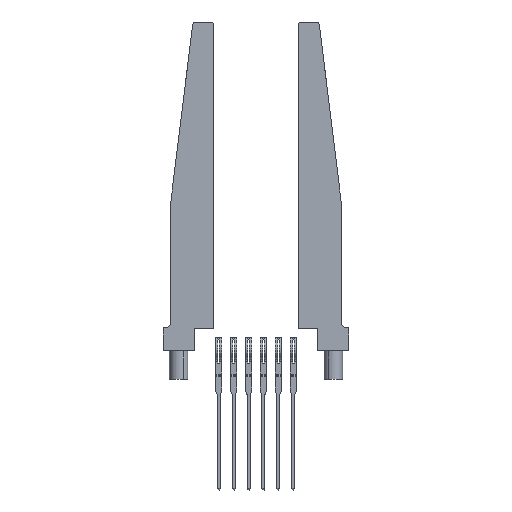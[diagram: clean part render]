
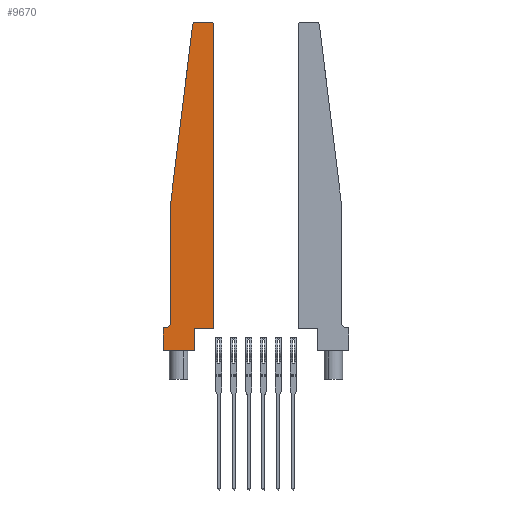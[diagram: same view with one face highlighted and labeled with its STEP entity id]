
A CAD part, top view. The second image highlights one B-rep face of the part: STEP entity #9670.
In plain terms, the highlighted planar face has unit normal (0, 0, 1).
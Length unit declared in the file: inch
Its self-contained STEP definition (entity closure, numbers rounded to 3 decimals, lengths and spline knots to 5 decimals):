
#51 = EDGE_CURVE ( 'NONE', #11635, #7275, #797, .T. ) ;
#185 = VECTOR ( 'NONE', #13633, 39.37008 ) ;
#228 = CARTESIAN_POINT ( 'NONE',  ( 0.065, 0.2375, 0.37 ) ) ;
#387 = CARTESIAN_POINT ( 'NONE',  ( 0.065, 1.25, 0.37 ) ) ;
#487 = VERTEX_POINT ( 'NONE', #6014 ) ;
#513 = DIRECTION ( 'NONE',  ( 0., 0., 1. ) ) ;
#551 = VERTEX_POINT ( 'NONE', #4396 ) ;
#700 = CARTESIAN_POINT ( 'NONE',  ( 0.015, 0.2375, 0.37 ) ) ;
#797 = LINE ( 'NONE', #8160, #4274 ) ;
#814 = ORIENTED_EDGE ( 'NONE', *, *, #6309, .T. ) ;
#1166 = CARTESIAN_POINT ( 'NONE',  ( 0.2605, 0.18, 0.37 ) ) ;
#1531 = EDGE_CURVE ( 'NONE', #5878, #4005, #7129, .T. ) ;
#1551 = EDGE_CURVE ( 'NONE', #8311, #2658, #11511, .T. ) ;
#1616 = CARTESIAN_POINT ( 'NONE',  ( 0.395, 2.75, 0.37 ) ) ;
#1831 = AXIS2_PLACEMENT_3D ( 'NONE', #700, #3854, #13475 ) ;
#1925 = DIRECTION ( 'NONE',  ( 1., 0., 0. ) ) ;
#1995 = CARTESIAN_POINT ( 'NONE',  ( 0., 0.1875, 0.37 ) ) ;
#2031 = DIRECTION ( 'NONE',  ( 1., 0., 0. ) ) ;
#2064 = FACE_OUTER_BOUND ( 'NONE', #13731, .T. ) ;
#2277 = VERTEX_POINT ( 'NONE', #7781 ) ;
#2502 = DIRECTION ( 'NONE',  ( 0., -1., 0. ) ) ;
#2549 = EDGE_CURVE ( 'NONE', #7275, #3619, #2656, .T. ) ;
#2588 = DIRECTION ( 'NONE',  ( 1., 0., 0. ) ) ;
#2656 = LINE ( 'NONE', #387, #12060 ) ;
#2658 = VERTEX_POINT ( 'NONE', #3944 ) ;
#2678 = VECTOR ( 'NONE', #10494, 39.37008 ) ;
#2684 = ORIENTED_EDGE ( 'NONE', *, *, #10316, .T. ) ;
#2731 = ORIENTED_EDGE ( 'NONE', *, *, #11652, .T. ) ;
#2940 = ORIENTED_EDGE ( 'NONE', *, *, #7992, .T. ) ;
#2974 = CARTESIAN_POINT ( 'NONE',  ( 0.25, 2.75, 0.37 ) ) ;
#3008 = VECTOR ( 'NONE', #7226, 39.37008 ) ;
#3022 = CARTESIAN_POINT ( 'NONE',  ( 0., 0., 0.37 ) ) ;
#3124 = CARTESIAN_POINT ( 'NONE',  ( 0.2605, 0.18, 0.37 ) ) ;
#3207 = ORIENTED_EDGE ( 'NONE', *, *, #13453, .T. ) ;
#3357 = LINE ( 'NONE', #1166, #5713 ) ;
#3521 = CARTESIAN_POINT ( 'NONE',  ( 0.425, 0.18, 0.37 ) ) ;
#3539 = DIRECTION ( 'NONE',  ( 0., -1., 0. ) ) ;
#3619 = VERTEX_POINT ( 'NONE', #228 ) ;
#3685 = ORIENTED_EDGE ( 'NONE', *, *, #2549, .T. ) ;
#3825 = EDGE_CURVE ( 'NONE', #9360, #8311, #7421, .T. ) ;
#3838 = CARTESIAN_POINT ( 'NONE',  ( 0.27653, 2.72, 0.37 ) ) ;
#3854 = DIRECTION ( 'NONE',  ( 0., 0., -1. ) ) ;
#3937 = CIRCLE ( 'NONE', #12690, 0.03 ) ;
#3944 = CARTESIAN_POINT ( 'NONE',  ( 0.425, 2.72, 0.37 ) ) ;
#4005 = VERTEX_POINT ( 'NONE', #13353 ) ;
#4274 = VECTOR ( 'NONE', #5124, 39.37008 ) ;
#4396 = CARTESIAN_POINT ( 'NONE',  ( 0.015, 0.1875, 0.37 ) ) ;
#4893 = ORIENTED_EDGE ( 'NONE', *, *, #3825, .T. ) ;
#5124 = DIRECTION ( 'NONE',  ( -0.122, -0.992, 0. ) ) ;
#5236 = CARTESIAN_POINT ( 'NONE',  ( 0.065, 0.1875, 0.37 ) ) ;
#5575 = ORIENTED_EDGE ( 'NONE', *, *, #1551, .T. ) ;
#5649 = EDGE_CURVE ( 'NONE', #487, #5951, #8904, .T. ) ;
#5713 = VECTOR ( 'NONE', #10914, 39.37008 ) ;
#5878 = VERTEX_POINT ( 'NONE', #1616 ) ;
#5951 = VERTEX_POINT ( 'NONE', #8202 ) ;
#6014 = CARTESIAN_POINT ( 'NONE',  ( 0., 0.1875, 0.37 ) ) ;
#6125 = EDGE_CURVE ( 'NONE', #4005, #11635, #10674, .T. ) ;
#6309 = EDGE_CURVE ( 'NONE', #3619, #551, #7946, .T. ) ;
#6326 = DIRECTION ( 'NONE',  ( 1., 0., 0. ) ) ;
#6698 = CARTESIAN_POINT ( 'NONE',  ( 0.065, 1.25, 0.37 ) ) ;
#6793 = DIRECTION ( 'NONE',  ( 0., 0., 1. ) ) ;
#7129 = LINE ( 'NONE', #2974, #2678 ) ;
#7226 = DIRECTION ( 'NONE',  ( -1., 0., 0. ) ) ;
#7275 = VERTEX_POINT ( 'NONE', #6698 ) ;
#7421 = LINE ( 'NONE', #8339, #8614 ) ;
#7781 = CARTESIAN_POINT ( 'NONE',  ( 0.2605, 0., 0.37 ) ) ;
#7946 = CIRCLE ( 'NONE', #1831, 0.05 ) ;
#7992 = EDGE_CURVE ( 'NONE', #5951, #2277, #11554, .T. ) ;
#8160 = CARTESIAN_POINT ( 'NONE',  ( 0.065, 1.25, 0.37 ) ) ;
#8202 = CARTESIAN_POINT ( 'NONE',  ( 0., 0., 0.37 ) ) ;
#8311 = VERTEX_POINT ( 'NONE', #3521 ) ;
#8339 = CARTESIAN_POINT ( 'NONE',  ( 0.425, 0.18, 0.37 ) ) ;
#8614 = VECTOR ( 'NONE', #2031, 39.37008 ) ;
#8662 = CARTESIAN_POINT ( 'NONE',  ( 0.24675, 2.72367, 0.37 ) ) ;
#8904 = LINE ( 'NONE', #13159, #11342 ) ;
#9291 = AXIS2_PLACEMENT_3D ( 'NONE', #3838, #6793, #11092 ) ;
#9297 = CARTESIAN_POINT ( 'NONE',  ( 0.425, 0.18, 0.37 ) ) ;
#9360 = VERTEX_POINT ( 'NONE', #3124 ) ;
#9670 = ADVANCED_FACE ( 'NONE', ( #2064 ), #10688, .T. ) ;
#10195 = AXIS2_PLACEMENT_3D ( 'NONE', #1995, #12708, #6326 ) ;
#10240 = VECTOR ( 'NONE', #1925, 39.37008 ) ;
#10316 = EDGE_CURVE ( 'NONE', #2658, #5878, #3937, .T. ) ;
#10494 = DIRECTION ( 'NONE',  ( -1., 0., 0. ) ) ;
#10590 = LINE ( 'NONE', #5236, #3008 ) ;
#10674 = CIRCLE ( 'NONE', #9291, 0.03 ) ;
#10688 = PLANE ( 'NONE',  #10195 ) ;
#10801 = ORIENTED_EDGE ( 'NONE', *, *, #5649, .T. ) ;
#10914 = DIRECTION ( 'NONE',  ( 0., 1., 0. ) ) ;
#11092 = DIRECTION ( 'NONE',  ( 1., 0., 0. ) ) ;
#11342 = VECTOR ( 'NONE', #3539, 39.37008 ) ;
#11511 = LINE ( 'NONE', #9297, #185 ) ;
#11554 = LINE ( 'NONE', #3022, #10240 ) ;
#11635 = VERTEX_POINT ( 'NONE', #8662 ) ;
#11652 = EDGE_CURVE ( 'NONE', #2277, #9360, #3357, .T. ) ;
#12060 = VECTOR ( 'NONE', #2502, 39.37008 ) ;
#12305 = CARTESIAN_POINT ( 'NONE',  ( 0.395, 2.72, 0.37 ) ) ;
#12690 = AXIS2_PLACEMENT_3D ( 'NONE', #12305, #513, #2588 ) ;
#12708 = DIRECTION ( 'NONE',  ( 0., 0., 1. ) ) ;
#13058 = ORIENTED_EDGE ( 'NONE', *, *, #6125, .T. ) ;
#13159 = CARTESIAN_POINT ( 'NONE',  ( 0., 0., 0.37 ) ) ;
#13353 = CARTESIAN_POINT ( 'NONE',  ( 0.27653, 2.75, 0.37 ) ) ;
#13374 = ORIENTED_EDGE ( 'NONE', *, *, #1531, .T. ) ;
#13453 = EDGE_CURVE ( 'NONE', #551, #487, #10590, .T. ) ;
#13475 = DIRECTION ( 'NONE',  ( -1., 0., 0. ) ) ;
#13633 = DIRECTION ( 'NONE',  ( 0., 1., 0. ) ) ;
#13731 = EDGE_LOOP ( 'NONE', ( #13374, #13058, #13741, #3685, #814, #3207, #10801, #2940, #2731, #4893, #5575, #2684 ) ) ;
#13741 = ORIENTED_EDGE ( 'NONE', *, *, #51, .T. ) ;
